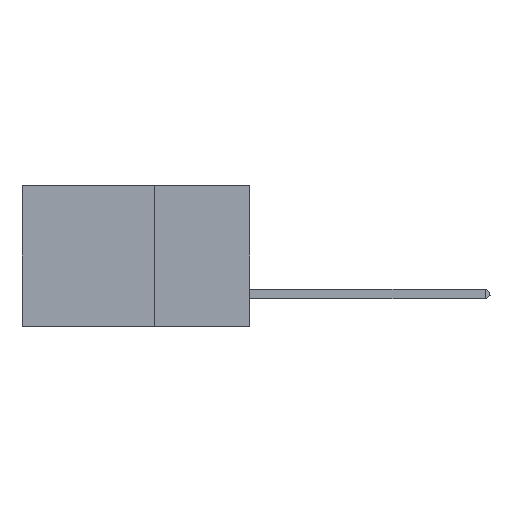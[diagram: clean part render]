
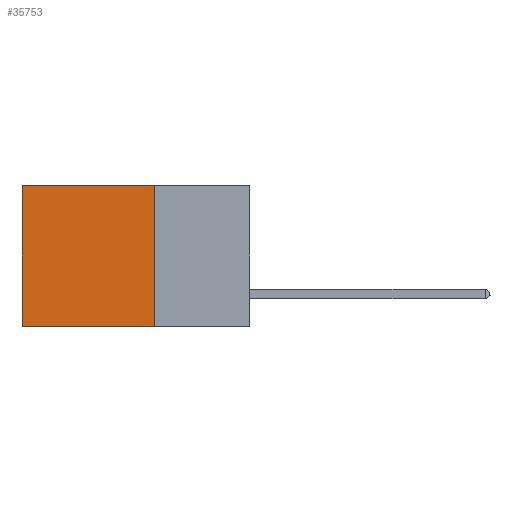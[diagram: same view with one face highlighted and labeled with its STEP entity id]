
A CAD part, left-side view. The second image highlights one B-rep face of the part: STEP entity #35753.
In plain terms, the highlighted planar face has unit normal (-1, 0, 0).
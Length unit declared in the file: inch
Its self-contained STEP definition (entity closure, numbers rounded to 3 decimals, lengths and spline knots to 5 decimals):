
#4485 = CARTESIAN_POINT ( 'NONE',  ( 0.2875, 0.25, 0. ) ) ;
#6150 = ORIENTED_EDGE ( 'NONE', *, *, #15374, .T. ) ;
#6729 = DIRECTION ( 'NONE',  ( 1., 0., 0. ) ) ;
#7947 = EDGE_CURVE ( 'NONE', #25671, #18907, #24194, .T. ) ;
#10544 = CARTESIAN_POINT ( 'NONE',  ( 0.2875, 0.25, -0.37 ) ) ;
#13227 = VERTEX_POINT ( 'NONE', #38668 ) ;
#14895 = LINE ( 'NONE', #40615, #28340 ) ;
#15374 = EDGE_CURVE ( 'NONE', #43514, #18907, #26899, .T. ) ;
#15756 = VECTOR ( 'NONE', #42025, 39.37008 ) ;
#16404 = EDGE_LOOP ( 'NONE', ( #6150, #29945, #21053, #33059 ) ) ;
#17804 = CARTESIAN_POINT ( 'NONE',  ( 0.2875, 0.6, 0. ) ) ;
#18002 = PLANE ( 'NONE',  #28480 ) ;
#18907 = VERTEX_POINT ( 'NONE', #19784 ) ;
#19784 = CARTESIAN_POINT ( 'NONE',  ( 0.2875, 0.6, -0.37 ) ) ;
#20714 = VECTOR ( 'NONE', #43600, 39.37008 ) ;
#21053 = ORIENTED_EDGE ( 'NONE', *, *, #37761, .F. ) ;
#22169 = LINE ( 'NONE', #4485, #15756 ) ;
#22231 = VECTOR ( 'NONE', #37423, 39.37008 ) ;
#24194 = LINE ( 'NONE', #28891, #20714 ) ;
#25671 = VERTEX_POINT ( 'NONE', #10544 ) ;
#26899 = LINE ( 'NONE', #44762, #22231 ) ;
#28340 = VECTOR ( 'NONE', #36900, 39.37008 ) ;
#28480 = AXIS2_PLACEMENT_3D ( 'NONE', #44119, #6729, #40352 ) ;
#28716 = EDGE_CURVE ( 'NONE', #13227, #43514, #22169, .T. ) ;
#28891 = CARTESIAN_POINT ( 'NONE',  ( 0.2875, 0.25, -0.37 ) ) ;
#29945 = ORIENTED_EDGE ( 'NONE', *, *, #7947, .F. ) ;
#33059 = ORIENTED_EDGE ( 'NONE', *, *, #28716, .T. ) ;
#33206 = FACE_OUTER_BOUND ( 'NONE', #16404, .T. ) ;
#35753 = ADVANCED_FACE ( 'NONE', ( #33206 ), #18002, .F. ) ;
#36900 = DIRECTION ( 'NONE',  ( 0., 0., -1. ) ) ;
#37423 = DIRECTION ( 'NONE',  ( 0., 0., -1. ) ) ;
#37761 = EDGE_CURVE ( 'NONE', #13227, #25671, #14895, .T. ) ;
#38668 = CARTESIAN_POINT ( 'NONE',  ( 0.2875, 0.25, 0. ) ) ;
#40352 = DIRECTION ( 'NONE',  ( 0., 0., -1. ) ) ;
#40615 = CARTESIAN_POINT ( 'NONE',  ( 0.2875, 0.25, 0. ) ) ;
#42025 = DIRECTION ( 'NONE',  ( 0., 1., 0. ) ) ;
#43514 = VERTEX_POINT ( 'NONE', #17804 ) ;
#43600 = DIRECTION ( 'NONE',  ( 0., 1., 0. ) ) ;
#44119 = CARTESIAN_POINT ( 'NONE',  ( 0.2875, 0.25, 0. ) ) ;
#44762 = CARTESIAN_POINT ( 'NONE',  ( 0.2875, 0.6, 0. ) ) ;
